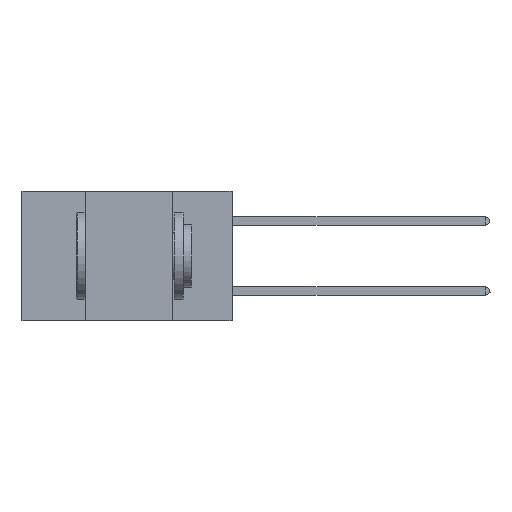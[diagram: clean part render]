
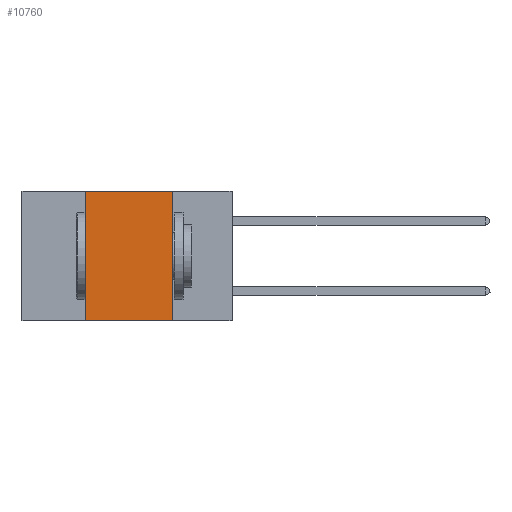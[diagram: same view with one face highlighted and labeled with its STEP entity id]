
A CAD part, left-side view. The second image highlights one B-rep face of the part: STEP entity #10760.
In plain terms, the highlighted planar face has unit normal (-1, 0, 0).
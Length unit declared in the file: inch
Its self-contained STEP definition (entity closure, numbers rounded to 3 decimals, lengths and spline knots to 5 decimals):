
#1192 = LINE ( 'NONE', #39888, #26351 ) ;
#1374 = DIRECTION ( 'NONE',  ( 0., 0., -1. ) ) ;
#1754 = AXIS2_PLACEMENT_3D ( 'NONE', #18756, #37733, #34492 ) ;
#5516 = EDGE_CURVE ( 'NONE', #37522, #26044, #1192, .T. ) ;
#7476 = DIRECTION ( 'NONE',  ( 0., 0., 1. ) ) ;
#7849 = CARTESIAN_POINT ( 'NONE',  ( 0., 0.42, -0.37 ) ) ;
#9875 = ORIENTED_EDGE ( 'NONE', *, *, #23144, .F. ) ;
#10760 = ADVANCED_FACE ( 'NONE', ( #40624 ), #18888, .F. ) ;
#18756 = CARTESIAN_POINT ( 'NONE',  ( 0., 0.6, 0. ) ) ;
#18888 = PLANE ( 'NONE',  #1754 ) ;
#20007 = CARTESIAN_POINT ( 'NONE',  ( 0., 0.17, 0. ) ) ;
#21139 = DIRECTION ( 'NONE',  ( 0., -1., 0. ) ) ;
#21302 = DIRECTION ( 'NONE',  ( 0., -1., 0. ) ) ;
#22600 = ORIENTED_EDGE ( 'NONE', *, *, #5516, .F. ) ;
#23144 = EDGE_CURVE ( 'NONE', #26044, #36037, #24479, .T. ) ;
#24149 = VERTEX_POINT ( 'NONE', #7849 ) ;
#24235 = EDGE_CURVE ( 'NONE', #24149, #36037, #35918, .T. ) ;
#24479 = LINE ( 'NONE', #27183, #35342 ) ;
#26044 = VERTEX_POINT ( 'NONE', #20007 ) ;
#26351 = VECTOR ( 'NONE', #21139, 39.37008 ) ;
#26890 = ORIENTED_EDGE ( 'NONE', *, *, #29446, .F. ) ;
#26926 = CARTESIAN_POINT ( 'NONE',  ( 0., 0.42, 0. ) ) ;
#27001 = VECTOR ( 'NONE', #21302, 39.37008 ) ;
#27007 = CARTESIAN_POINT ( 'NONE',  ( 0., 0.42, 0. ) ) ;
#27183 = CARTESIAN_POINT ( 'NONE',  ( 0., 0.17, 0. ) ) ;
#29140 = EDGE_LOOP ( 'NONE', ( #9875, #22600, #26890, #34468 ) ) ;
#29446 = EDGE_CURVE ( 'NONE', #24149, #37522, #36845, .T. ) ;
#30244 = CARTESIAN_POINT ( 'NONE',  ( 0., 0.17, -0.37 ) ) ;
#34351 = CARTESIAN_POINT ( 'NONE',  ( 0., 0.6, -0.37 ) ) ;
#34468 = ORIENTED_EDGE ( 'NONE', *, *, #24235, .T. ) ;
#34492 = DIRECTION ( 'NONE',  ( 0., 0., -1. ) ) ;
#35342 = VECTOR ( 'NONE', #1374, 39.37008 ) ;
#35918 = LINE ( 'NONE', #34351, #27001 ) ;
#36037 = VERTEX_POINT ( 'NONE', #30244 ) ;
#36845 = LINE ( 'NONE', #26926, #38805 ) ;
#37522 = VERTEX_POINT ( 'NONE', #27007 ) ;
#37733 = DIRECTION ( 'NONE',  ( 1., 0., 0. ) ) ;
#38805 = VECTOR ( 'NONE', #7476, 39.37008 ) ;
#39888 = CARTESIAN_POINT ( 'NONE',  ( 0., 0.6, 0. ) ) ;
#40624 = FACE_OUTER_BOUND ( 'NONE', #29140, .T. ) ;
